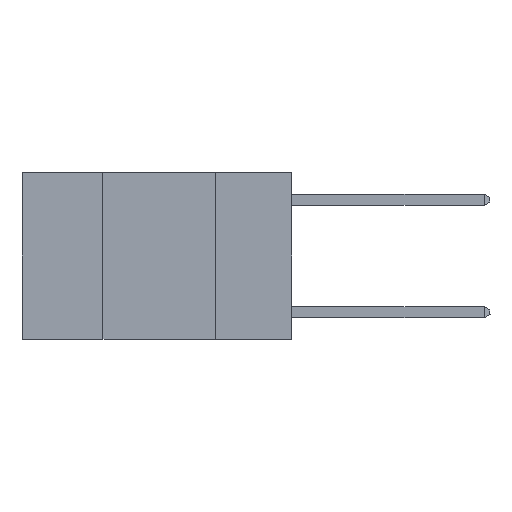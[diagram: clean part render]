
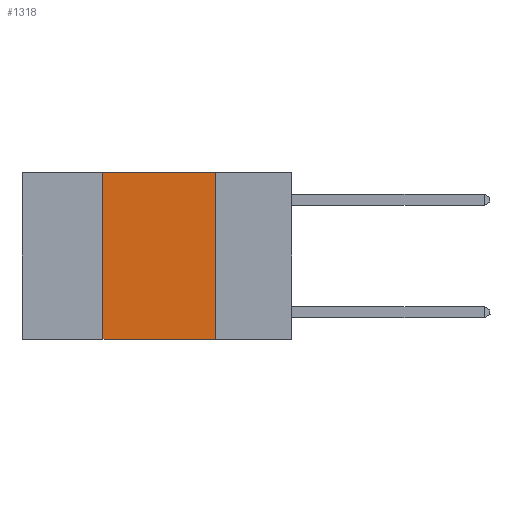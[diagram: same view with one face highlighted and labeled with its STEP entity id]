
A CAD part, left-side view. The second image highlights one B-rep face of the part: STEP entity #1318.
In plain terms, the highlighted planar face has unit normal (-1, 0, 0).
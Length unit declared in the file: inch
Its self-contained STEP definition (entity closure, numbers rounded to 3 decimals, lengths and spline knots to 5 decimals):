
#836 = VERTEX_POINT ( 'NONE', #8686 ) ;
#1318 = ADVANCED_FACE ( 'NONE', ( #18699 ), #18032, .F. ) ;
#1406 = CARTESIAN_POINT ( 'NONE',  ( 0., 0.6, 0. ) ) ;
#2316 = VECTOR ( 'NONE', #3680, 39.37008 ) ;
#2924 = CARTESIAN_POINT ( 'NONE',  ( 0., 0.17, 0. ) ) ;
#3091 = DIRECTION ( 'NONE',  ( 0., -1., 0. ) ) ;
#3615 = DIRECTION ( 'NONE',  ( 0., 0., 1. ) ) ;
#3680 = DIRECTION ( 'NONE',  ( 0., -1., 0. ) ) ;
#6224 = EDGE_CURVE ( 'NONE', #18231, #836, #25439, .T. ) ;
#7186 = DIRECTION ( 'NONE',  ( 0., 0., -1. ) ) ;
#7458 = CARTESIAN_POINT ( 'NONE',  ( 0., 0.6, -0.37 ) ) ;
#8686 = CARTESIAN_POINT ( 'NONE',  ( 0., 0.17, -0.37 ) ) ;
#9258 = CARTESIAN_POINT ( 'NONE',  ( 0., 0.42, -0.37 ) ) ;
#9793 = LINE ( 'NONE', #7458, #14735 ) ;
#10124 = ORIENTED_EDGE ( 'NONE', *, *, #6224, .F. ) ;
#10846 = EDGE_LOOP ( 'NONE', ( #10124, #26917, #16390, #27560 ) ) ;
#11617 = VERTEX_POINT ( 'NONE', #9258 ) ;
#11877 = EDGE_CURVE ( 'NONE', #11617, #17815, #24185, .T. ) ;
#13703 = LINE ( 'NONE', #1406, #2316 ) ;
#14043 = CARTESIAN_POINT ( 'NONE',  ( 0., 0.42, 0. ) ) ;
#14735 = VECTOR ( 'NONE', #3091, 39.37008 ) ;
#15109 = DIRECTION ( 'NONE',  ( 0., 0., -1. ) ) ;
#15594 = CARTESIAN_POINT ( 'NONE',  ( 0., 0.17, 0. ) ) ;
#15651 = DIRECTION ( 'NONE',  ( 1., 0., 0. ) ) ;
#16390 = ORIENTED_EDGE ( 'NONE', *, *, #11877, .F. ) ;
#17034 = CARTESIAN_POINT ( 'NONE',  ( 0., 0.6, 0. ) ) ;
#17815 = VERTEX_POINT ( 'NONE', #14043 ) ;
#18032 = PLANE ( 'NONE',  #20316 ) ;
#18231 = VERTEX_POINT ( 'NONE', #2924 ) ;
#18699 = FACE_OUTER_BOUND ( 'NONE', #10846, .T. ) ;
#18971 = EDGE_CURVE ( 'NONE', #11617, #836, #9793, .T. ) ;
#19839 = VECTOR ( 'NONE', #7186, 39.37008 ) ;
#20316 = AXIS2_PLACEMENT_3D ( 'NONE', #17034, #15651, #15109 ) ;
#23511 = VECTOR ( 'NONE', #3615, 39.37008 ) ;
#24185 = LINE ( 'NONE', #26836, #23511 ) ;
#25439 = LINE ( 'NONE', #15594, #19839 ) ;
#26836 = CARTESIAN_POINT ( 'NONE',  ( 0., 0.42, 0. ) ) ;
#26917 = ORIENTED_EDGE ( 'NONE', *, *, #27237, .F. ) ;
#27237 = EDGE_CURVE ( 'NONE', #17815, #18231, #13703, .T. ) ;
#27560 = ORIENTED_EDGE ( 'NONE', *, *, #18971, .T. ) ;
